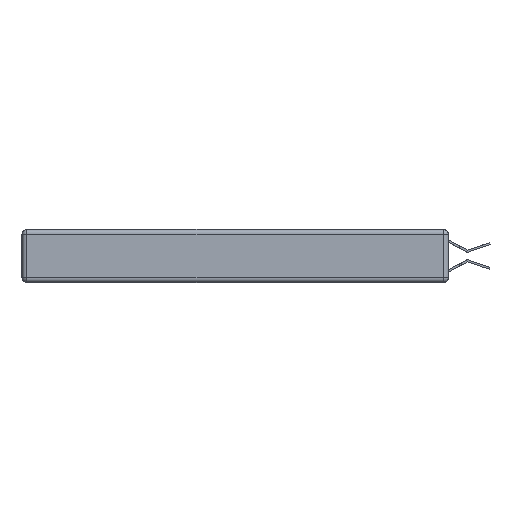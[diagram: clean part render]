
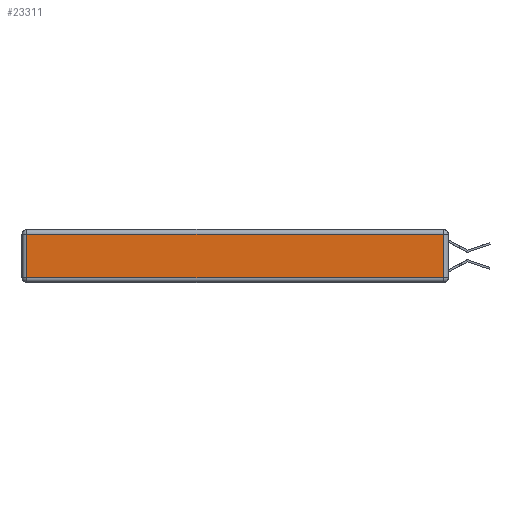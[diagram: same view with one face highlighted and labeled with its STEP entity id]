
A CAD part, left-side view. The second image highlights one B-rep face of the part: STEP entity #23311.
In plain terms, the highlighted planar face has unit normal (-1, 0, 0).
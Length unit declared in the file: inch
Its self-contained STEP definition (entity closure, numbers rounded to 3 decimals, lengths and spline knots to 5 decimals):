
#153 = EDGE_CURVE ( 'NONE', #15357, #24367, #25122, .T. ) ;
#842 = CARTESIAN_POINT ( 'NONE',  ( 0., 2.72, -0.343 ) ) ;
#1196 = VECTOR ( 'NONE', #13036, 39.37008 ) ;
#2328 = CARTESIAN_POINT ( 'NONE',  ( 0., 0., -0.343 ) ) ;
#2407 = EDGE_CURVE ( 'NONE', #24367, #19976, #6209, .T. ) ;
#3803 = LINE ( 'NONE', #4775, #25579 ) ;
#4730 = ORIENTED_EDGE ( 'NONE', *, *, #7588, .T. ) ;
#4775 = CARTESIAN_POINT ( 'NONE',  ( 0., 2.75, -0.03 ) ) ;
#5170 = FACE_OUTER_BOUND ( 'NONE', #16811, .T. ) ;
#5481 = CARTESIAN_POINT ( 'NONE',  ( 0., 2.72, -0.313 ) ) ;
#5944 = CARTESIAN_POINT ( 'NONE',  ( 0., 0.03, -0.03 ) ) ;
#6209 = LINE ( 'NONE', #7053, #1196 ) ;
#6882 = EDGE_CURVE ( 'NONE', #19976, #19603, #3803, .T. ) ;
#7053 = CARTESIAN_POINT ( 'NONE',  ( 0., 0.03, -0.343 ) ) ;
#7166 = CARTESIAN_POINT ( 'NONE',  ( 0., 0., -0.313 ) ) ;
#7588 = EDGE_CURVE ( 'NONE', #19603, #15357, #20488, .T. ) ;
#8326 = ORIENTED_EDGE ( 'NONE', *, *, #153, .T. ) ;
#8786 = VECTOR ( 'NONE', #14944, 39.37008 ) ;
#13036 = DIRECTION ( 'NONE',  ( 0., 0., 1. ) ) ;
#14655 = DIRECTION ( 'NONE',  ( 0., 0., 1. ) ) ;
#14909 = DIRECTION ( 'NONE',  ( 0., 1., 0. ) ) ;
#14944 = DIRECTION ( 'NONE',  ( 0., 0., -1. ) ) ;
#15357 = VERTEX_POINT ( 'NONE', #5481 ) ;
#16591 = ORIENTED_EDGE ( 'NONE', *, *, #6882, .T. ) ;
#16811 = EDGE_LOOP ( 'NONE', ( #8326, #20392, #16591, #4730 ) ) ;
#17213 = VECTOR ( 'NONE', #19336, 39.37008 ) ;
#18455 = PLANE ( 'NONE',  #23707 ) ;
#19336 = DIRECTION ( 'NONE',  ( 0., -1., 0. ) ) ;
#19603 = VERTEX_POINT ( 'NONE', #22705 ) ;
#19976 = VERTEX_POINT ( 'NONE', #5944 ) ;
#20392 = ORIENTED_EDGE ( 'NONE', *, *, #2407, .T. ) ;
#20488 = LINE ( 'NONE', #842, #8786 ) ;
#20495 = DIRECTION ( 'NONE',  ( -1., 0., 0. ) ) ;
#22705 = CARTESIAN_POINT ( 'NONE',  ( 0., 2.72, -0.03 ) ) ;
#23311 = ADVANCED_FACE ( 'NONE', ( #5170 ), #18455, .T. ) ;
#23418 = CARTESIAN_POINT ( 'NONE',  ( 0., 0.03, -0.313 ) ) ;
#23707 = AXIS2_PLACEMENT_3D ( 'NONE', #2328, #20495, #14655 ) ;
#24367 = VERTEX_POINT ( 'NONE', #23418 ) ;
#25122 = LINE ( 'NONE', #7166, #17213 ) ;
#25579 = VECTOR ( 'NONE', #14909, 39.37008 ) ;
